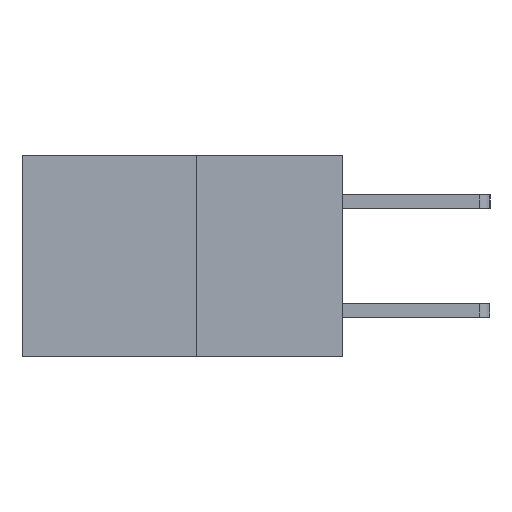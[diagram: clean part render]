
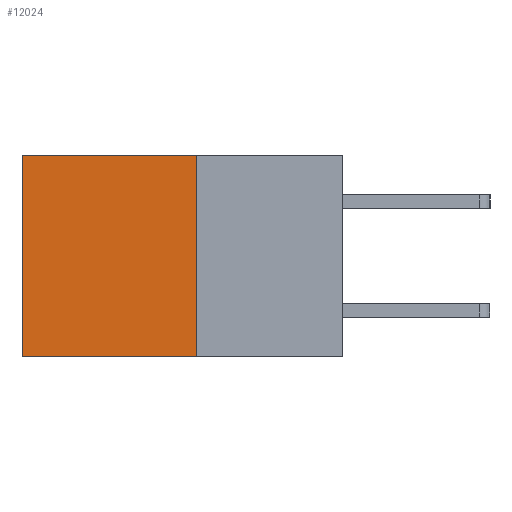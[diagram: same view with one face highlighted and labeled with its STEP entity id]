
A CAD part, left-side view. The second image highlights one B-rep face of the part: STEP entity #12024.
In plain terms, the highlighted planar face has unit normal (-1, 0, 0).
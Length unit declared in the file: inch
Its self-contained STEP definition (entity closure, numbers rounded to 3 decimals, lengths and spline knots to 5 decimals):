
#128 = CARTESIAN_POINT ( 'NONE',  ( 0.277, 0.27, 0. ) ) ;
#412 = ORIENTED_EDGE ( 'NONE', *, *, #2285, .F. ) ;
#753 = ORIENTED_EDGE ( 'NONE', *, *, #9695, .T. ) ;
#1145 = EDGE_LOOP ( 'NONE', ( #10054, #2223, #412, #753 ) ) ;
#1460 = VECTOR ( 'NONE', #12163, 39.37008 ) ;
#1506 = LINE ( 'NONE', #4589, #11942 ) ;
#1680 = CARTESIAN_POINT ( 'NONE',  ( 0.277, 0.59, -0.37 ) ) ;
#1947 = VECTOR ( 'NONE', #11434, 39.37008 ) ;
#2014 = VECTOR ( 'NONE', #9849, 39.37008 ) ;
#2210 = CARTESIAN_POINT ( 'NONE',  ( 0.277, 0.59, -0.37 ) ) ;
#2223 = ORIENTED_EDGE ( 'NONE', *, *, #3699, .F. ) ;
#2285 = EDGE_CURVE ( 'NONE', #10902, #6748, #12364, .T. ) ;
#3387 = AXIS2_PLACEMENT_3D ( 'NONE', #5284, #12292, #6301 ) ;
#3699 = EDGE_CURVE ( 'NONE', #6748, #4436, #7211, .T. ) ;
#4035 = FACE_OUTER_BOUND ( 'NONE', #1145, .T. ) ;
#4436 = VERTEX_POINT ( 'NONE', #2210 ) ;
#4589 = CARTESIAN_POINT ( 'NONE',  ( 0.277, 0.27, 0. ) ) ;
#5284 = CARTESIAN_POINT ( 'NONE',  ( 0.277, 0.27, -0.37 ) ) ;
#5603 = DIRECTION ( 'NONE',  ( 0., 1., 0. ) ) ;
#5671 = CARTESIAN_POINT ( 'NONE',  ( 0.277, 0.59, 0. ) ) ;
#6170 = CARTESIAN_POINT ( 'NONE',  ( 0.277, 0.27, -0.37 ) ) ;
#6301 = DIRECTION ( 'NONE',  ( 0., 0., -1. ) ) ;
#6748 = VERTEX_POINT ( 'NONE', #9243 ) ;
#7211 = LINE ( 'NONE', #6170, #1460 ) ;
#7458 = LINE ( 'NONE', #1680, #2014 ) ;
#8463 = EDGE_CURVE ( 'NONE', #10443, #4436, #7458, .T. ) ;
#9243 = CARTESIAN_POINT ( 'NONE',  ( 0.277, 0.27, -0.37 ) ) ;
#9695 = EDGE_CURVE ( 'NONE', #10902, #10443, #1506, .T. ) ;
#9849 = DIRECTION ( 'NONE',  ( 0., 0., -1. ) ) ;
#10054 = ORIENTED_EDGE ( 'NONE', *, *, #8463, .T. ) ;
#10443 = VERTEX_POINT ( 'NONE', #5671 ) ;
#10902 = VERTEX_POINT ( 'NONE', #128 ) ;
#11200 = CARTESIAN_POINT ( 'NONE',  ( 0.277, 0.27, -0.37 ) ) ;
#11325 = PLANE ( 'NONE',  #3387 ) ;
#11434 = DIRECTION ( 'NONE',  ( 0., 0., -1. ) ) ;
#11942 = VECTOR ( 'NONE', #5603, 39.37008 ) ;
#12024 = ADVANCED_FACE ( 'NONE', ( #4035 ), #11325, .F. ) ;
#12163 = DIRECTION ( 'NONE',  ( 0., 1., 0. ) ) ;
#12292 = DIRECTION ( 'NONE',  ( 1., 0., 0. ) ) ;
#12364 = LINE ( 'NONE', #11200, #1947 ) ;
